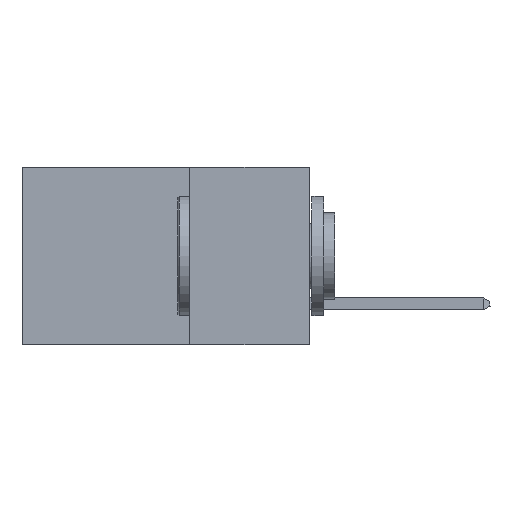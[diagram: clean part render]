
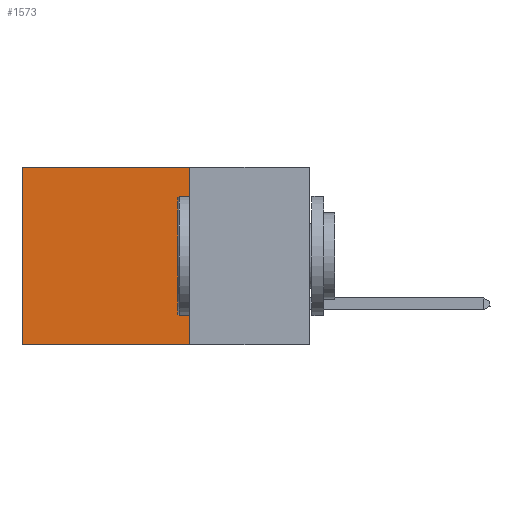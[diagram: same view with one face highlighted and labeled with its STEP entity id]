
A CAD part, left-side view. The second image highlights one B-rep face of the part: STEP entity #1573.
In plain terms, the highlighted planar face has unit normal (-1, 0, 0).
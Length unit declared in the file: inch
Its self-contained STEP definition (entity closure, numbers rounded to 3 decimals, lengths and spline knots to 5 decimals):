
#558 = CARTESIAN_POINT ( 'NONE',  ( 0.2875, 0.6, 0. ) ) ;
#1041 = CARTESIAN_POINT ( 'NONE',  ( 0.2875, 0.25, -0.37 ) ) ;
#1425 = DIRECTION ( 'NONE',  ( 1., 0., 0. ) ) ;
#1573 = ADVANCED_FACE ( 'NONE', ( #17320 ), #12864, .F. ) ;
#1951 = ORIENTED_EDGE ( 'NONE', *, *, #24020, .F. ) ;
#2001 = CARTESIAN_POINT ( 'NONE',  ( 0.2875, 0.25, 0. ) ) ;
#2455 = CARTESIAN_POINT ( 'NONE',  ( 0.2875, 0.6, -0.37 ) ) ;
#3107 = AXIS2_PLACEMENT_3D ( 'NONE', #24266, #1425, #14523 ) ;
#4279 = VERTEX_POINT ( 'NONE', #7788 ) ;
#4473 = EDGE_CURVE ( 'NONE', #16279, #22489, #11501, .T. ) ;
#5364 = ORIENTED_EDGE ( 'NONE', *, *, #6780, .T. ) ;
#5403 = ORIENTED_EDGE ( 'NONE', *, *, #4473, .F. ) ;
#6574 = ORIENTED_EDGE ( 'NONE', *, *, #11627, .T. ) ;
#6780 = EDGE_CURVE ( 'NONE', #4279, #10172, #13014, .T. ) ;
#7601 = VECTOR ( 'NONE', #19349, 39.37008 ) ;
#7788 = CARTESIAN_POINT ( 'NONE',  ( 0.2875, 0.25, 0. ) ) ;
#10172 = VERTEX_POINT ( 'NONE', #11585 ) ;
#11501 = LINE ( 'NONE', #1041, #15661 ) ;
#11585 = CARTESIAN_POINT ( 'NONE',  ( 0.2875, 0.6, 0. ) ) ;
#11627 = EDGE_CURVE ( 'NONE', #10172, #22489, #17863, .T. ) ;
#12030 = EDGE_LOOP ( 'NONE', ( #6574, #5403, #1951, #5364 ) ) ;
#12864 = PLANE ( 'NONE',  #3107 ) ;
#13014 = LINE ( 'NONE', #2001, #7601 ) ;
#14523 = DIRECTION ( 'NONE',  ( 0., 0., -1. ) ) ;
#15661 = VECTOR ( 'NONE', #20513, 39.37008 ) ;
#16279 = VERTEX_POINT ( 'NONE', #18645 ) ;
#16671 = VECTOR ( 'NONE', #21898, 39.37008 ) ;
#17320 = FACE_OUTER_BOUND ( 'NONE', #12030, .T. ) ;
#17863 = LINE ( 'NONE', #558, #16671 ) ;
#18645 = CARTESIAN_POINT ( 'NONE',  ( 0.2875, 0.25, -0.37 ) ) ;
#19349 = DIRECTION ( 'NONE',  ( 0., 1., 0. ) ) ;
#19702 = VECTOR ( 'NONE', #23458, 39.37008 ) ;
#20513 = DIRECTION ( 'NONE',  ( 0., 1., 0. ) ) ;
#21522 = CARTESIAN_POINT ( 'NONE',  ( 0.2875, 0.25, 0. ) ) ;
#21898 = DIRECTION ( 'NONE',  ( 0., 0., -1. ) ) ;
#22489 = VERTEX_POINT ( 'NONE', #2455 ) ;
#23039 = LINE ( 'NONE', #21522, #19702 ) ;
#23458 = DIRECTION ( 'NONE',  ( 0., 0., -1. ) ) ;
#24020 = EDGE_CURVE ( 'NONE', #4279, #16279, #23039, .T. ) ;
#24266 = CARTESIAN_POINT ( 'NONE',  ( 0.2875, 0.25, 0. ) ) ;
